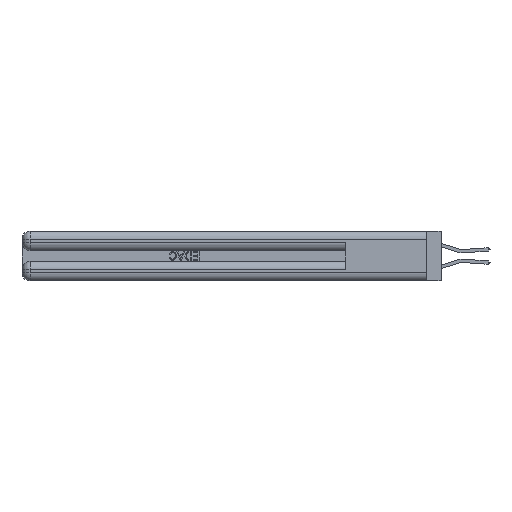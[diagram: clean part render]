
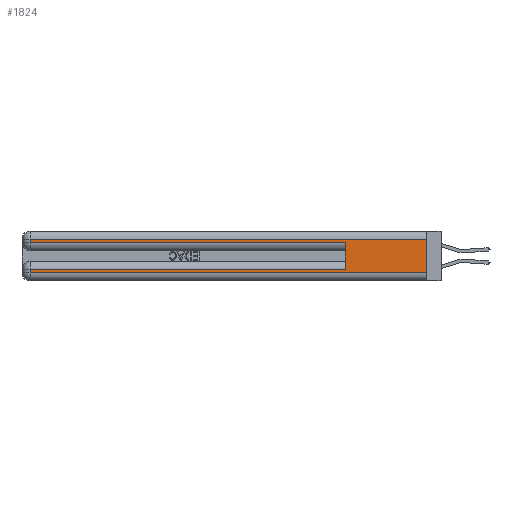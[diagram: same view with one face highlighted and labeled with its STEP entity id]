
A CAD part, left-side view. The second image highlights one B-rep face of the part: STEP entity #1824.
In plain terms, the highlighted planar face has unit normal (-1, 0, 0).
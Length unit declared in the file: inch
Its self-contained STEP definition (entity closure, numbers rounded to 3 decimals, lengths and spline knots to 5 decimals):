
#343 = VECTOR ( 'NONE', #31243, 39.37008 ) ;
#707 = VERTEX_POINT ( 'NONE', #1063 ) ;
#1063 = CARTESIAN_POINT ( 'NONE',  ( 0., 0.6, 0.085 ) ) ;
#1264 = VERTEX_POINT ( 'NONE', #4975 ) ;
#1582 = CARTESIAN_POINT ( 'NONE',  ( 0., 0., 0.37 ) ) ;
#1824 = ADVANCED_FACE ( 'NONE', ( #17819 ), #41299, .F. ) ;
#2010 = CARTESIAN_POINT ( 'NONE',  ( 0., 2.94, 0.37 ) ) ;
#2094 = DIRECTION ( 'NONE',  ( 0., 1., 0. ) ) ;
#2213 = VERTEX_POINT ( 'NONE', #27008 ) ;
#2488 = VECTOR ( 'NONE', #41389, 39.37008 ) ;
#4975 = CARTESIAN_POINT ( 'NONE',  ( 0., 0.6, 0.285 ) ) ;
#5541 = LINE ( 'NONE', #38259, #12296 ) ;
#6022 = VECTOR ( 'NONE', #2094, 39.37008 ) ;
#6937 = LINE ( 'NONE', #2010, #39019 ) ;
#8284 = DIRECTION ( 'NONE',  ( 1., 0., 0. ) ) ;
#8484 = AXIS2_PLACEMENT_3D ( 'NONE', #1582, #8284, #25186 ) ;
#8523 = CARTESIAN_POINT ( 'NONE',  ( 0., 0., 0.285 ) ) ;
#9006 = DIRECTION ( 'NONE',  ( 0., 0., -1. ) ) ;
#9069 = EDGE_CURVE ( 'NONE', #27494, #1264, #22213, .T. ) ;
#10190 = VECTOR ( 'NONE', #20815, 39.37008 ) ;
#10847 = CARTESIAN_POINT ( 'NONE',  ( 0., 2.94, 0.31 ) ) ;
#11100 = VECTOR ( 'NONE', #34880, 39.37008 ) ;
#11484 = EDGE_CURVE ( 'NONE', #35567, #2213, #5541, .T. ) ;
#12228 = EDGE_CURVE ( 'NONE', #13377, #28323, #42778, .T. ) ;
#12296 = VECTOR ( 'NONE', #19149, 39.37008 ) ;
#13162 = LINE ( 'NONE', #34977, #11100 ) ;
#13377 = VERTEX_POINT ( 'NONE', #30723 ) ;
#14819 = ORIENTED_EDGE ( 'NONE', *, *, #41907, .F. ) ;
#15600 = ORIENTED_EDGE ( 'NONE', *, *, #34838, .T. ) ;
#16926 = VECTOR ( 'NONE', #42105, 39.37008 ) ;
#17819 = FACE_OUTER_BOUND ( 'NONE', #26902, .T. ) ;
#18164 = ORIENTED_EDGE ( 'NONE', *, *, #12228, .T. ) ;
#18304 = EDGE_CURVE ( 'NONE', #707, #1264, #36550, .T. ) ;
#18597 = CARTESIAN_POINT ( 'NONE',  ( 0., 0., 0.37 ) ) ;
#19149 = DIRECTION ( 'NONE',  ( 0., -1., 0. ) ) ;
#20815 = DIRECTION ( 'NONE',  ( 0., 0., 1. ) ) ;
#22213 = LINE ( 'NONE', #8523, #2488 ) ;
#22843 = VERTEX_POINT ( 'NONE', #24700 ) ;
#24700 = CARTESIAN_POINT ( 'NONE',  ( 0., 2.94, 0.085 ) ) ;
#25186 = DIRECTION ( 'NONE',  ( 0., 0., -1. ) ) ;
#25544 = CARTESIAN_POINT ( 'NONE',  ( 0., 0., 0.31 ) ) ;
#26902 = EDGE_LOOP ( 'NONE', ( #14819, #18164, #15600, #42397, #28515, #33278, #28808, #37905 ) ) ;
#27008 = CARTESIAN_POINT ( 'NONE',  ( 0., 0., 0.06 ) ) ;
#27494 = VERTEX_POINT ( 'NONE', #35235 ) ;
#27832 = LINE ( 'NONE', #18597, #16926 ) ;
#27860 = LINE ( 'NONE', #38056, #343 ) ;
#28323 = VERTEX_POINT ( 'NONE', #10847 ) ;
#28515 = ORIENTED_EDGE ( 'NONE', *, *, #18304, .F. ) ;
#28808 = ORIENTED_EDGE ( 'NONE', *, *, #34776, .T. ) ;
#30723 = CARTESIAN_POINT ( 'NONE',  ( 0., 0., 0.31 ) ) ;
#30939 = CARTESIAN_POINT ( 'NONE',  ( 0., 0.6, 0.145 ) ) ;
#31243 = DIRECTION ( 'NONE',  ( 0., 1., 0. ) ) ;
#33278 = ORIENTED_EDGE ( 'NONE', *, *, #42901, .T. ) ;
#34776 = EDGE_CURVE ( 'NONE', #22843, #35567, #13162, .T. ) ;
#34838 = EDGE_CURVE ( 'NONE', #28323, #27494, #6937, .T. ) ;
#34880 = DIRECTION ( 'NONE',  ( 0., 0., -1. ) ) ;
#34977 = CARTESIAN_POINT ( 'NONE',  ( 0., 2.94, 0.37 ) ) ;
#35235 = CARTESIAN_POINT ( 'NONE',  ( 0., 2.94, 0.285 ) ) ;
#35567 = VERTEX_POINT ( 'NONE', #35840 ) ;
#35840 = CARTESIAN_POINT ( 'NONE',  ( 0., 2.94, 0.06 ) ) ;
#36550 = LINE ( 'NONE', #30939, #10190 ) ;
#37905 = ORIENTED_EDGE ( 'NONE', *, *, #11484, .T. ) ;
#38056 = CARTESIAN_POINT ( 'NONE',  ( 0., 0., 0.085 ) ) ;
#38259 = CARTESIAN_POINT ( 'NONE',  ( 0., 0., 0.06 ) ) ;
#39019 = VECTOR ( 'NONE', #9006, 39.37008 ) ;
#41299 = PLANE ( 'NONE',  #8484 ) ;
#41389 = DIRECTION ( 'NONE',  ( 0., -1., 0. ) ) ;
#41907 = EDGE_CURVE ( 'NONE', #13377, #2213, #27832, .T. ) ;
#42105 = DIRECTION ( 'NONE',  ( 0., 0., -1. ) ) ;
#42397 = ORIENTED_EDGE ( 'NONE', *, *, #9069, .T. ) ;
#42778 = LINE ( 'NONE', #25544, #6022 ) ;
#42901 = EDGE_CURVE ( 'NONE', #707, #22843, #27860, .T. ) ;
